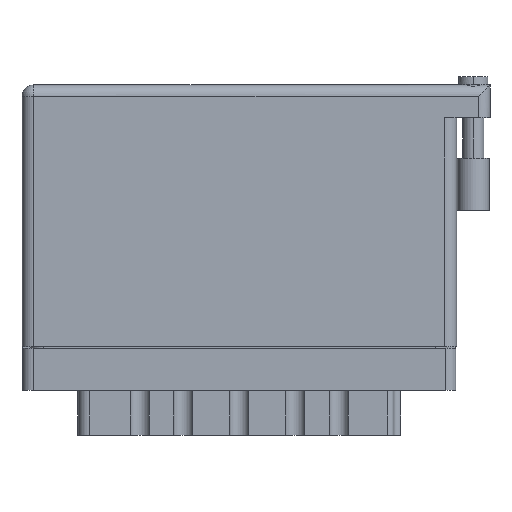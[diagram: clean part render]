
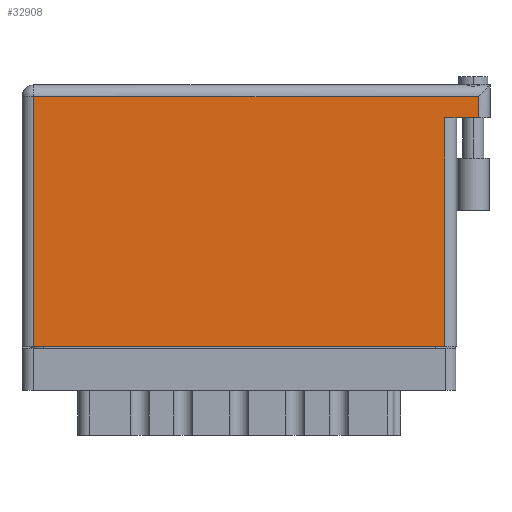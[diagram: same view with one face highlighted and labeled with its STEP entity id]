
A CAD part, front view. The second image highlights one B-rep face of the part: STEP entity #32908.
In plain terms, the highlighted face is planar.
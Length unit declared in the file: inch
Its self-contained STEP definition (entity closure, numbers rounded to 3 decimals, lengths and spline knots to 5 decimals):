
#360 = VERTEX_POINT ( 'NONE', #50849 ) ;
#999 = VECTOR ( 'NONE', #15617, 39.37008 ) ;
#1084 = DIRECTION ( 'NONE',  ( 0., 1., 0. ) ) ;
#3164 = DIRECTION ( 'NONE',  ( 0., 1., 0. ) ) ;
#4489 = LINE ( 'NONE', #38206, #46929 ) ;
#4721 = VERTEX_POINT ( 'NONE', #51988 ) ;
#7955 = VECTOR ( 'NONE', #1084, 39.37008 ) ;
#8035 = ORIENTED_EDGE ( 'NONE', *, *, #35110, .T. ) ;
#9620 = VECTOR ( 'NONE', #53046, 39.37008 ) ;
#11003 = CARTESIAN_POINT ( 'NONE',  ( 0., 1.566, 0. ) ) ;
#11048 = EDGE_CURVE ( 'NONE', #51015, #23603, #26813, .T. ) ;
#11628 = ORIENTED_EDGE ( 'NONE', *, *, #52513, .F. ) ;
#13347 = EDGE_CURVE ( 'NONE', #23603, #51494, #29768, .T. ) ;
#13661 = LINE ( 'NONE', #23620, #49109 ) ;
#13902 = DIRECTION ( 'NONE',  ( -1., 0., 0. ) ) ;
#15617 = DIRECTION ( 'NONE',  ( -1., 0., 0. ) ) ;
#16360 = LINE ( 'NONE', #23733, #999 ) ;
#17171 = VECTOR ( 'NONE', #18649, 39.37008 ) ;
#17775 = EDGE_CURVE ( 'NONE', #4721, #21882, #13661, .T. ) ;
#18649 = DIRECTION ( 'NONE',  ( 1., 0., 0. ) ) ;
#20552 = LINE ( 'NONE', #43159, #9620 ) ;
#21882 = VERTEX_POINT ( 'NONE', #22943 ) ;
#22943 = CARTESIAN_POINT ( 'NONE',  ( 2.73, 1.496, 0. ) ) ;
#23603 = VERTEX_POINT ( 'NONE', #24609 ) ;
#23620 = CARTESIAN_POINT ( 'NONE',  ( 2.73, 1.566, 0. ) ) ;
#23733 = CARTESIAN_POINT ( 'NONE',  ( 0., 1.496, 0. ) ) ;
#24609 = CARTESIAN_POINT ( 'NONE',  ( 2.53, 0., 0. ) ) ;
#25649 = CARTESIAN_POINT ( 'NONE',  ( 2.53, 1.369, 0. ) ) ;
#26506 = ORIENTED_EDGE ( 'NONE', *, *, #13347, .T. ) ;
#26509 = ORIENTED_EDGE ( 'NONE', *, *, #42952, .T. ) ;
#26813 = LINE ( 'NONE', #34865, #17171 ) ;
#29768 = LINE ( 'NONE', #50874, #7955 ) ;
#31842 = PLANE ( 'NONE',  #43090 ) ;
#32908 = ADVANCED_FACE ( 'NONE', ( #49390 ), #31842, .F. ) ;
#34865 = CARTESIAN_POINT ( 'NONE',  ( 0., 0., 0. ) ) ;
#35110 = EDGE_CURVE ( 'NONE', #21882, #360, #16360, .T. ) ;
#36183 = DIRECTION ( 'NONE',  ( 0., 0., -1. ) ) ;
#37506 = ORIENTED_EDGE ( 'NONE', *, *, #17775, .T. ) ;
#38206 = CARTESIAN_POINT ( 'NONE',  ( 2.8, 1.369, 0. ) ) ;
#42952 = EDGE_CURVE ( 'NONE', #360, #51015, #20552, .T. ) ;
#43090 = AXIS2_PLACEMENT_3D ( 'NONE', #11003, #36183, #52597 ) ;
#43159 = CARTESIAN_POINT ( 'NONE',  ( 0.07, 0., 0. ) ) ;
#44708 = EDGE_LOOP ( 'NONE', ( #48072, #26506, #11628, #37506, #8035, #26509 ) ) ;
#46247 = CARTESIAN_POINT ( 'NONE',  ( 0.07, 0., 0. ) ) ;
#46929 = VECTOR ( 'NONE', #13902, 39.37008 ) ;
#48072 = ORIENTED_EDGE ( 'NONE', *, *, #11048, .T. ) ;
#49109 = VECTOR ( 'NONE', #3164, 39.37008 ) ;
#49390 = FACE_OUTER_BOUND ( 'NONE', #44708, .T. ) ;
#50849 = CARTESIAN_POINT ( 'NONE',  ( 0.07, 1.496, 0. ) ) ;
#50874 = CARTESIAN_POINT ( 'NONE',  ( 2.53, 1.369, 0. ) ) ;
#51015 = VERTEX_POINT ( 'NONE', #46247 ) ;
#51494 = VERTEX_POINT ( 'NONE', #25649 ) ;
#51988 = CARTESIAN_POINT ( 'NONE',  ( 2.73, 1.369, 0. ) ) ;
#52513 = EDGE_CURVE ( 'NONE', #4721, #51494, #4489, .T. ) ;
#52597 = DIRECTION ( 'NONE',  ( -1., 0., 0. ) ) ;
#53046 = DIRECTION ( 'NONE',  ( 0., -1., 0. ) ) ;
